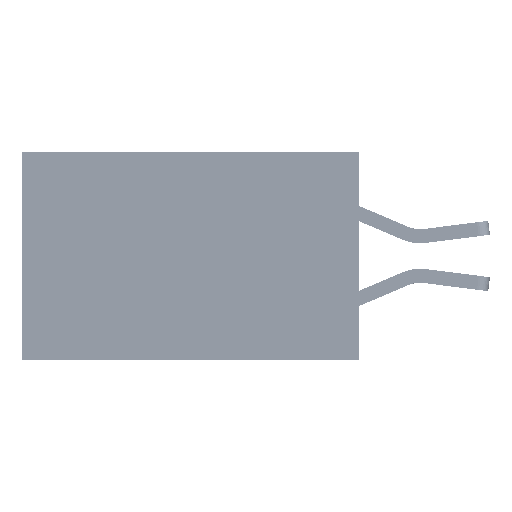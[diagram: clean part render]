
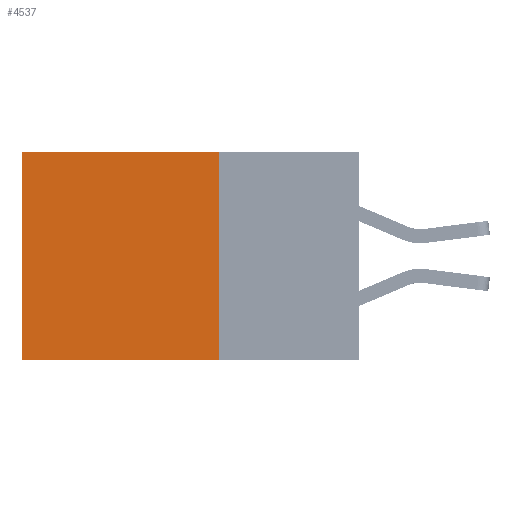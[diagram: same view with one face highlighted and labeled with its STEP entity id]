
A CAD part, left-side view. The second image highlights one B-rep face of the part: STEP entity #4537.
In plain terms, the highlighted planar face has unit normal (-1, 0, 0).
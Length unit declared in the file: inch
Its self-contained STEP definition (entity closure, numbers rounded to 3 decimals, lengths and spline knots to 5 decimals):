
#73 = VERTEX_POINT ( 'NONE', #12899 ) ;
#534 = CARTESIAN_POINT ( 'NONE',  ( 0.2875, 0.6, 0. ) ) ;
#1517 = PLANE ( 'NONE',  #8588 ) ;
#1608 = DIRECTION ( 'NONE',  ( 0., 0., -1. ) ) ;
#3004 = VECTOR ( 'NONE', #1608, 39.37008 ) ;
#3201 = CARTESIAN_POINT ( 'NONE',  ( 0.2875, 0.6, 0. ) ) ;
#3540 = VECTOR ( 'NONE', #26940, 39.37008 ) ;
#4537 = ADVANCED_FACE ( 'NONE', ( #17560 ), #1517, .F. ) ;
#4764 = LINE ( 'NONE', #37906, #5310 ) ;
#4985 = VERTEX_POINT ( 'NONE', #534 ) ;
#5310 = VECTOR ( 'NONE', #41865, 39.37008 ) ;
#5744 = EDGE_LOOP ( 'NONE', ( #45067, #30504, #9814, #31763 ) ) ;
#6356 = CARTESIAN_POINT ( 'NONE',  ( 0.2875, 0.25, 0. ) ) ;
#8588 = AXIS2_PLACEMENT_3D ( 'NONE', #9099, #19396, #44715 ) ;
#9099 = CARTESIAN_POINT ( 'NONE',  ( 0.2875, 0.25, 0. ) ) ;
#9814 = ORIENTED_EDGE ( 'NONE', *, *, #13686, .F. ) ;
#9857 = VECTOR ( 'NONE', #17126, 39.37008 ) ;
#12899 = CARTESIAN_POINT ( 'NONE',  ( 0.2875, 0.25, 0. ) ) ;
#13686 = EDGE_CURVE ( 'NONE', #73, #23437, #4764, .T. ) ;
#17126 = DIRECTION ( 'NONE',  ( 0., 1., 0. ) ) ;
#17560 = FACE_OUTER_BOUND ( 'NONE', #5744, .T. ) ;
#18807 = EDGE_CURVE ( 'NONE', #23437, #26005, #27797, .T. ) ;
#19396 = DIRECTION ( 'NONE',  ( 1., 0., 0. ) ) ;
#23437 = VERTEX_POINT ( 'NONE', #41355 ) ;
#26005 = VERTEX_POINT ( 'NONE', #45319 ) ;
#26940 = DIRECTION ( 'NONE',  ( 0., 1., 0. ) ) ;
#27100 = CARTESIAN_POINT ( 'NONE',  ( 0.2875, 0.25, -0.37 ) ) ;
#27797 = LINE ( 'NONE', #27100, #3540 ) ;
#30504 = ORIENTED_EDGE ( 'NONE', *, *, #18807, .F. ) ;
#31763 = ORIENTED_EDGE ( 'NONE', *, *, #31967, .T. ) ;
#31967 = EDGE_CURVE ( 'NONE', #73, #4985, #37559, .T. ) ;
#36448 = LINE ( 'NONE', #3201, #3004 ) ;
#37559 = LINE ( 'NONE', #6356, #9857 ) ;
#37906 = CARTESIAN_POINT ( 'NONE',  ( 0.2875, 0.25, 0. ) ) ;
#41036 = EDGE_CURVE ( 'NONE', #4985, #26005, #36448, .T. ) ;
#41355 = CARTESIAN_POINT ( 'NONE',  ( 0.2875, 0.25, -0.37 ) ) ;
#41865 = DIRECTION ( 'NONE',  ( 0., 0., -1. ) ) ;
#44715 = DIRECTION ( 'NONE',  ( 0., 0., -1. ) ) ;
#45067 = ORIENTED_EDGE ( 'NONE', *, *, #41036, .T. ) ;
#45319 = CARTESIAN_POINT ( 'NONE',  ( 0.2875, 0.6, -0.37 ) ) ;
